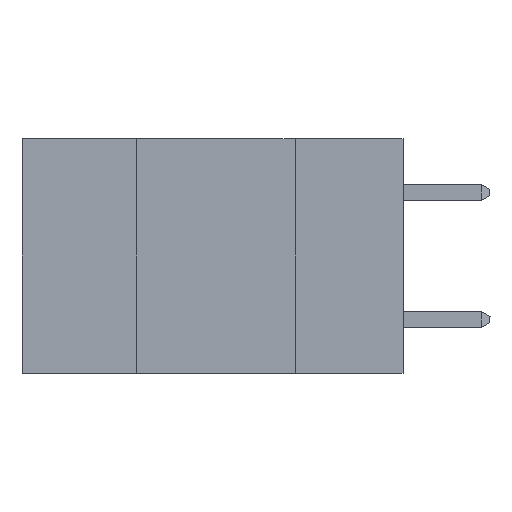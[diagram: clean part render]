
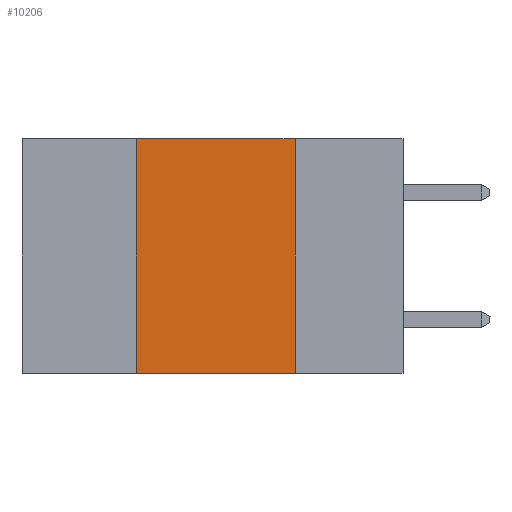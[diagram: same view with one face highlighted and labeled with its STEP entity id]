
A CAD part, left-side view. The second image highlights one B-rep face of the part: STEP entity #10206.
In plain terms, the highlighted planar face has unit normal (-1, 0, 0).
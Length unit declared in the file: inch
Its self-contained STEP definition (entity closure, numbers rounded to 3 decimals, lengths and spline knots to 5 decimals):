
#2765 = ORIENTED_EDGE ( 'NONE', *, *, #15812, .T. ) ;
#2892 = DIRECTION ( 'NONE',  ( 0., -1., 0. ) ) ;
#4033 = VECTOR ( 'NONE', #17425, 39.37008 ) ;
#4505 = CARTESIAN_POINT ( 'NONE',  ( 0., 0.17, 0. ) ) ;
#4544 = VERTEX_POINT ( 'NONE', #8220 ) ;
#4646 = EDGE_CURVE ( 'NONE', #17044, #10651, #20778, .T. ) ;
#5735 = CARTESIAN_POINT ( 'NONE',  ( 0., 0.6, 0. ) ) ;
#5862 = VECTOR ( 'NONE', #19647, 39.37008 ) ;
#6819 = CARTESIAN_POINT ( 'NONE',  ( 0., 0.42, 0. ) ) ;
#7409 = DIRECTION ( 'NONE',  ( 0., 0., -1. ) ) ;
#8220 = CARTESIAN_POINT ( 'NONE',  ( 0., 0.42, -0.37 ) ) ;
#8735 = ORIENTED_EDGE ( 'NONE', *, *, #18613, .F. ) ;
#8837 = CARTESIAN_POINT ( 'NONE',  ( 0., 0.6, 0. ) ) ;
#10206 = ADVANCED_FACE ( 'NONE', ( #14224 ), #14213, .F. ) ;
#10651 = VERTEX_POINT ( 'NONE', #10968 ) ;
#10968 = CARTESIAN_POINT ( 'NONE',  ( 0., 0.17, -0.37 ) ) ;
#11191 = ORIENTED_EDGE ( 'NONE', *, *, #4646, .F. ) ;
#11577 = VERTEX_POINT ( 'NONE', #20831 ) ;
#12892 = CARTESIAN_POINT ( 'NONE',  ( 0., 0.17, 0. ) ) ;
#13290 = LINE ( 'NONE', #5735, #5862 ) ;
#14213 = PLANE ( 'NONE',  #20345 ) ;
#14224 = FACE_OUTER_BOUND ( 'NONE', #20387, .T. ) ;
#14330 = ORIENTED_EDGE ( 'NONE', *, *, #14562, .F. ) ;
#14562 = EDGE_CURVE ( 'NONE', #4544, #11577, #18891, .T. ) ;
#15360 = CARTESIAN_POINT ( 'NONE',  ( 0., 0.6, -0.37 ) ) ;
#15812 = EDGE_CURVE ( 'NONE', #4544, #10651, #17564, .T. ) ;
#16099 = VECTOR ( 'NONE', #7409, 39.37008 ) ;
#17044 = VERTEX_POINT ( 'NONE', #4505 ) ;
#17425 = DIRECTION ( 'NONE',  ( 0., 0., 1. ) ) ;
#17564 = LINE ( 'NONE', #15360, #22221 ) ;
#18613 = EDGE_CURVE ( 'NONE', #11577, #17044, #13290, .T. ) ;
#18891 = LINE ( 'NONE', #6819, #4033 ) ;
#19416 = DIRECTION ( 'NONE',  ( 1., 0., 0. ) ) ;
#19492 = DIRECTION ( 'NONE',  ( 0., 0., -1. ) ) ;
#19647 = DIRECTION ( 'NONE',  ( 0., -1., 0. ) ) ;
#20345 = AXIS2_PLACEMENT_3D ( 'NONE', #8837, #19416, #19492 ) ;
#20387 = EDGE_LOOP ( 'NONE', ( #11191, #8735, #14330, #2765 ) ) ;
#20778 = LINE ( 'NONE', #12892, #16099 ) ;
#20831 = CARTESIAN_POINT ( 'NONE',  ( 0., 0.42, 0. ) ) ;
#22221 = VECTOR ( 'NONE', #2892, 39.37008 ) ;
